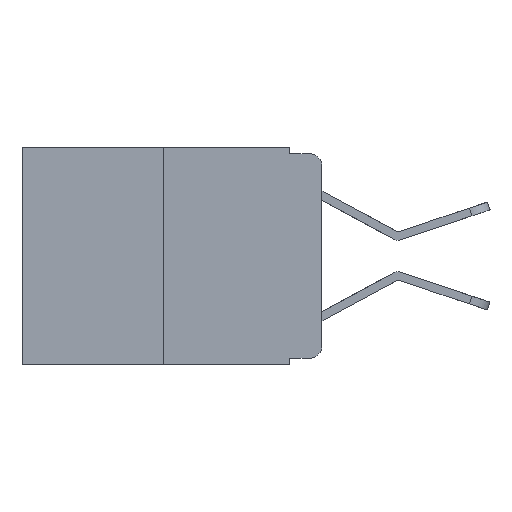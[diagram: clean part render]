
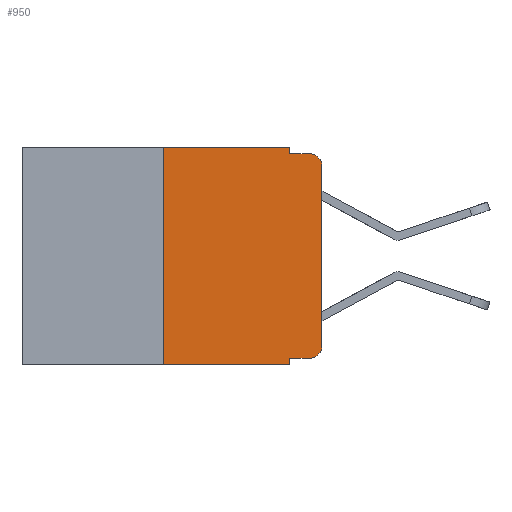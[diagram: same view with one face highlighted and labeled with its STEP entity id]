
A CAD part, left-side view. The second image highlights one B-rep face of the part: STEP entity #950.
In plain terms, the highlighted planar face has unit normal (-1, 0, 0).
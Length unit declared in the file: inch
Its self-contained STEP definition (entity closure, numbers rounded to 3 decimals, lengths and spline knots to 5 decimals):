
#19 = CARTESIAN_POINT ( 'NONE',  ( 0., 0.473, -0.343 ) ) ;
#79 = CARTESIAN_POINT ( 'NONE',  ( 0., 0.02, -0.333 ) ) ;
#88 = AXIS2_PLACEMENT_3D ( 'NONE', #6595, #1617, #7376 ) ;
#119 = CARTESIAN_POINT ( 'NONE',  ( 0., 0.02, -0.01 ) ) ;
#640 = DIRECTION ( 'NONE',  ( 1., 0., 0. ) ) ;
#686 = ORIENTED_EDGE ( 'NONE', *, *, #9754, .F. ) ;
#950 = ADVANCED_FACE ( 'NONE', ( #2848 ), #9923, .F. ) ;
#975 = LINE ( 'NONE', #9154, #7304 ) ;
#1104 = CARTESIAN_POINT ( 'NONE',  ( 0., 0.051, 0. ) ) ;
#1154 = DIRECTION ( 'NONE',  ( 0., -1., 0. ) ) ;
#1200 = ORIENTED_EDGE ( 'NONE', *, *, #9686, .F. ) ;
#1288 = CARTESIAN_POINT ( 'NONE',  ( 0., 0.473, 0. ) ) ;
#1341 = CARTESIAN_POINT ( 'NONE',  ( 0., 0.02, -0.03 ) ) ;
#1471 = ORIENTED_EDGE ( 'NONE', *, *, #9055, .T. ) ;
#1543 = VERTEX_POINT ( 'NONE', #2156 ) ;
#1545 = VERTEX_POINT ( 'NONE', #2102 ) ;
#1617 = DIRECTION ( 'NONE',  ( -1., 0., 0. ) ) ;
#1621 = DIRECTION ( 'NONE',  ( 0., -1., 0. ) ) ;
#1714 = VERTEX_POINT ( 'NONE', #4806 ) ;
#1822 = VECTOR ( 'NONE', #6352, 39.37008 ) ;
#1909 = DIRECTION ( 'NONE',  ( 0., 0., -1. ) ) ;
#2102 = CARTESIAN_POINT ( 'NONE',  ( 0., 0.051, -0.01 ) ) ;
#2137 = VECTOR ( 'NONE', #6918, 39.37008 ) ;
#2156 = CARTESIAN_POINT ( 'NONE',  ( 0., 0.051, -0.333 ) ) ;
#2206 = DIRECTION ( 'NONE',  ( 0., 0., -1. ) ) ;
#2216 = CARTESIAN_POINT ( 'NONE',  ( 0., 0.051, -0.343 ) ) ;
#2486 = EDGE_CURVE ( 'NONE', #1543, #6753, #5683, .T. ) ;
#2505 = CARTESIAN_POINT ( 'NONE',  ( 0., 0.25, 0. ) ) ;
#2567 = VERTEX_POINT ( 'NONE', #3899 ) ;
#2601 = VERTEX_POINT ( 'NONE', #8853 ) ;
#2618 = EDGE_CURVE ( 'NONE', #1543, #7603, #9056, .T. ) ;
#2745 = EDGE_LOOP ( 'NONE', ( #7997, #1471, #5669, #1200, #5189, #686, #10306, #6277, #5555, #3066 ) ) ;
#2848 = FACE_OUTER_BOUND ( 'NONE', #2745, .T. ) ;
#3053 = CARTESIAN_POINT ( 'NONE',  ( 0., 0.473, 0. ) ) ;
#3066 = ORIENTED_EDGE ( 'NONE', *, *, #10042, .T. ) ;
#3120 = EDGE_CURVE ( 'NONE', #1545, #5994, #4955, .T. ) ;
#3430 = CARTESIAN_POINT ( 'NONE',  ( 0., 0.051, 0. ) ) ;
#3899 = CARTESIAN_POINT ( 'NONE',  ( 0., 0.25, -0.343 ) ) ;
#4095 = LINE ( 'NONE', #6263, #1822 ) ;
#4140 = AXIS2_PLACEMENT_3D ( 'NONE', #1288, #640, #8121 ) ;
#4165 = VECTOR ( 'NONE', #6173, 39.37008 ) ;
#4398 = VECTOR ( 'NONE', #1154, 39.37008 ) ;
#4806 = CARTESIAN_POINT ( 'NONE',  ( 0., 0., -0.03 ) ) ;
#4955 = LINE ( 'NONE', #9341, #4398 ) ;
#5013 = EDGE_CURVE ( 'NONE', #2601, #1714, #4095, .T. ) ;
#5189 = ORIENTED_EDGE ( 'NONE', *, *, #5449, .F. ) ;
#5449 = EDGE_CURVE ( 'NONE', #5636, #8808, #6007, .T. ) ;
#5492 = VECTOR ( 'NONE', #6397, 39.37008 ) ;
#5555 = ORIENTED_EDGE ( 'NONE', *, *, #2618, .T. ) ;
#5636 = VERTEX_POINT ( 'NONE', #2505 ) ;
#5669 = ORIENTED_EDGE ( 'NONE', *, *, #3120, .F. ) ;
#5683 = LINE ( 'NONE', #1104, #9528 ) ;
#5932 = EDGE_CURVE ( 'NONE', #2567, #6753, #7583, .T. ) ;
#5994 = VERTEX_POINT ( 'NONE', #119 ) ;
#6007 = LINE ( 'NONE', #3053, #9598 ) ;
#6088 = CIRCLE ( 'NONE', #6917, 0.02 ) ;
#6173 = DIRECTION ( 'NONE',  ( 0., 0., 1. ) ) ;
#6263 = CARTESIAN_POINT ( 'NONE',  ( 0., 0., 0. ) ) ;
#6277 = ORIENTED_EDGE ( 'NONE', *, *, #2486, .F. ) ;
#6307 = LINE ( 'NONE', #6971, #4165 ) ;
#6352 = DIRECTION ( 'NONE',  ( 0., 0., 1. ) ) ;
#6397 = DIRECTION ( 'NONE',  ( 0., -1., 0. ) ) ;
#6595 = CARTESIAN_POINT ( 'NONE',  ( 0., 0.02, -0.313 ) ) ;
#6627 = DIRECTION ( 'NONE',  ( 0., 0., -1. ) ) ;
#6753 = VERTEX_POINT ( 'NONE', #2216 ) ;
#6917 = AXIS2_PLACEMENT_3D ( 'NONE', #1341, #7132, #2206 ) ;
#6918 = DIRECTION ( 'NONE',  ( 0., -1., 0. ) ) ;
#6971 = CARTESIAN_POINT ( 'NONE',  ( 0., 0.25, 0. ) ) ;
#7132 = DIRECTION ( 'NONE',  ( -1., 0., 0. ) ) ;
#7304 = VECTOR ( 'NONE', #1909, 39.37008 ) ;
#7376 = DIRECTION ( 'NONE',  ( 0., 0., -1. ) ) ;
#7530 = CIRCLE ( 'NONE', #88, 0.02 ) ;
#7583 = LINE ( 'NONE', #19, #5492 ) ;
#7603 = VERTEX_POINT ( 'NONE', #79 ) ;
#7997 = ORIENTED_EDGE ( 'NONE', *, *, #5013, .T. ) ;
#8121 = DIRECTION ( 'NONE',  ( 0., 0., -1. ) ) ;
#8439 = CARTESIAN_POINT ( 'NONE',  ( 0., 0.051, -0.333 ) ) ;
#8808 = VERTEX_POINT ( 'NONE', #3430 ) ;
#8853 = CARTESIAN_POINT ( 'NONE',  ( 0., 0., -0.313 ) ) ;
#9055 = EDGE_CURVE ( 'NONE', #1714, #5994, #6088, .T. ) ;
#9056 = LINE ( 'NONE', #8439, #2137 ) ;
#9154 = CARTESIAN_POINT ( 'NONE',  ( 0., 0.051, 0. ) ) ;
#9341 = CARTESIAN_POINT ( 'NONE',  ( 0., 0.051, -0.01 ) ) ;
#9528 = VECTOR ( 'NONE', #6627, 39.37008 ) ;
#9598 = VECTOR ( 'NONE', #1621, 39.37008 ) ;
#9686 = EDGE_CURVE ( 'NONE', #8808, #1545, #975, .T. ) ;
#9754 = EDGE_CURVE ( 'NONE', #2567, #5636, #6307, .T. ) ;
#9923 = PLANE ( 'NONE',  #4140 ) ;
#10042 = EDGE_CURVE ( 'NONE', #7603, #2601, #7530, .T. ) ;
#10306 = ORIENTED_EDGE ( 'NONE', *, *, #5932, .T. ) ;
